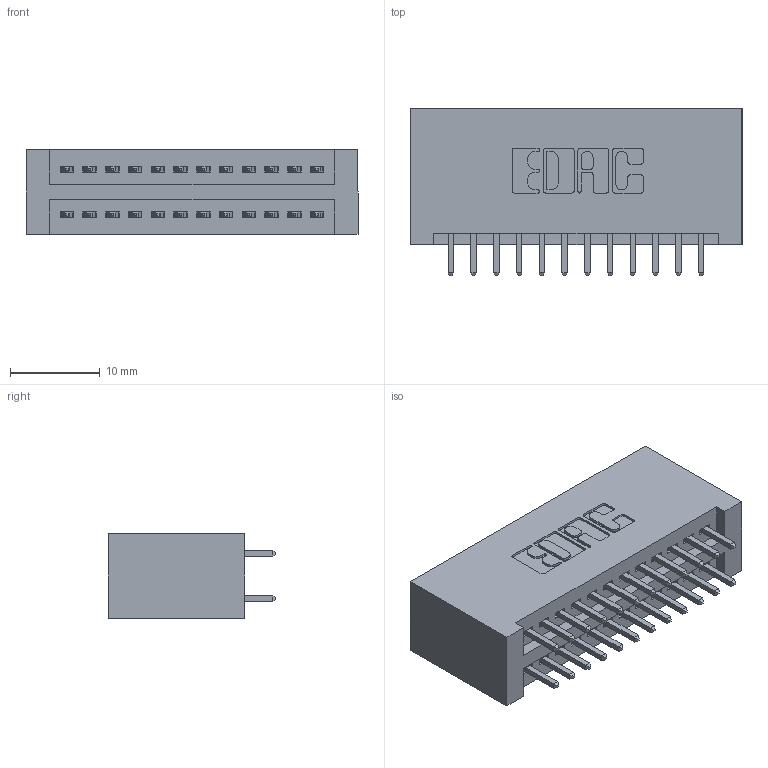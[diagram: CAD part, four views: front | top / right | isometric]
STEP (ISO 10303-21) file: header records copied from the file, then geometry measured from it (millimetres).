
FILE_DESCRIPTION (( 'STEP AP203' ), '1' );
FILE_NAME ('345-024-521-201.STEP', '2019-10-27T16:25:49', ( '' ), ( '' ), 'SwSTEP 2.0', 'SolidWorks 2016', '' );
FILE_SCHEMA (( 'CONFIG_CONTROL_DESIGN' ));
Length unit declared in the file: inch
Products named in the file (3): 345 Part_No Mounting Lugs; 345-292-001_345-293-121; 345-024-521-201
Assembly tree (25 placements, depth 2):
  345-024-521-201
    345 Part_No Mounting Lugs
    345-292-001_345-293-121  x24
Bounding box: 37.08 x 18.72 x 9.4 mm (x, y, z)
Volume: 3930 mm3; surface area: 5467.7 mm2
Topology: 25 solids, 25 shells, 1318 faces, 3893 edges, 2562 vertices
Faces by surface type: plane 868, cylinder 450
Entity records: 13195 total; most frequent: CARTESIAN_POINT 2240, ORIENTED_EDGE 2174, DIRECTION 2007, EDGE_CURVE 1087, VECTOR 915, LINE 915, VERTEX_POINT 722, AXIS2_PLACEMENT_3D 546
